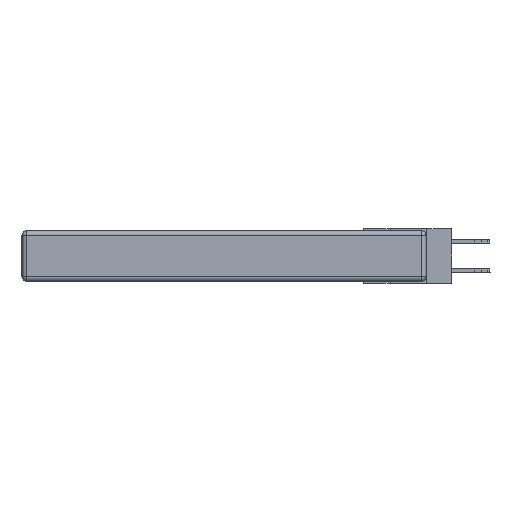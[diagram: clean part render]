
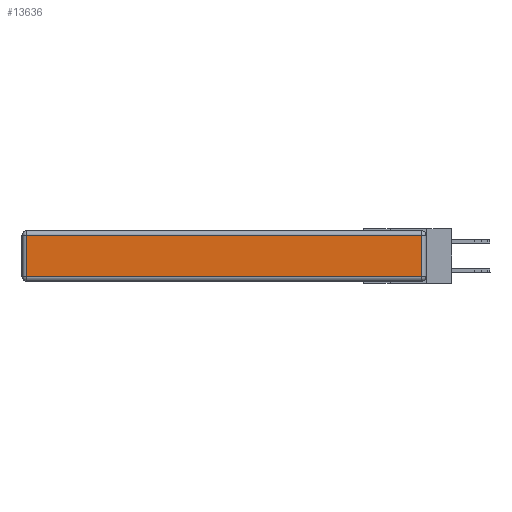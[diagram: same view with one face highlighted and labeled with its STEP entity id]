
A CAD part, left-side view. The second image highlights one B-rep face of the part: STEP entity #13636.
In plain terms, the highlighted planar face has unit normal (-1, 0, 0).
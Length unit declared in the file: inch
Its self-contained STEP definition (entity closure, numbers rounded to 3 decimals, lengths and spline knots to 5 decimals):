
#1110 = CARTESIAN_POINT ( 'NONE',  ( 0., 0.03, -0.313 ) ) ;
#1272 = CARTESIAN_POINT ( 'NONE',  ( 0., 0., -0.343 ) ) ;
#2018 = ORIENTED_EDGE ( 'NONE', *, *, #2638, .T. ) ;
#2610 = VECTOR ( 'NONE', #11376, 39.37008 ) ;
#2638 = EDGE_CURVE ( 'NONE', #4004, #21221, #9904, .T. ) ;
#3493 = VECTOR ( 'NONE', #21026, 39.37008 ) ;
#3643 = CARTESIAN_POINT ( 'NONE',  ( 0., 2.72, -0.313 ) ) ;
#4004 = VERTEX_POINT ( 'NONE', #5706 ) ;
#5398 = AXIS2_PLACEMENT_3D ( 'NONE', #1272, #11630, #13740 ) ;
#5706 = CARTESIAN_POINT ( 'NONE',  ( 0., 0.03, -0.03 ) ) ;
#6139 = DIRECTION ( 'NONE',  ( 0., -1., 0. ) ) ;
#6244 = PLANE ( 'NONE',  #5398 ) ;
#8753 = CARTESIAN_POINT ( 'NONE',  ( 0., 2.72, -0.03 ) ) ;
#9904 = LINE ( 'NONE', #11605, #2610 ) ;
#9993 = LINE ( 'NONE', #13917, #16485 ) ;
#10216 = LINE ( 'NONE', #13760, #3493 ) ;
#10365 = EDGE_LOOP ( 'NONE', ( #19891, #15674, #2018, #19196 ) ) ;
#10647 = FACE_OUTER_BOUND ( 'NONE', #10365, .T. ) ;
#11045 = LINE ( 'NONE', #13548, #17545 ) ;
#11376 = DIRECTION ( 'NONE',  ( 0., 1., 0. ) ) ;
#11605 = CARTESIAN_POINT ( 'NONE',  ( 0., 2.75, -0.03 ) ) ;
#11630 = DIRECTION ( 'NONE',  ( -1., 0., 0. ) ) ;
#11913 = EDGE_CURVE ( 'NONE', #21221, #13949, #10216, .T. ) ;
#12049 = DIRECTION ( 'NONE',  ( 0., 0., 1. ) ) ;
#12522 = EDGE_CURVE ( 'NONE', #13949, #19612, #11045, .T. ) ;
#13548 = CARTESIAN_POINT ( 'NONE',  ( 0., 0., -0.313 ) ) ;
#13636 = ADVANCED_FACE ( 'NONE', ( #10647 ), #6244, .T. ) ;
#13740 = DIRECTION ( 'NONE',  ( 0., 0., 1. ) ) ;
#13760 = CARTESIAN_POINT ( 'NONE',  ( 0., 2.72, -0.343 ) ) ;
#13917 = CARTESIAN_POINT ( 'NONE',  ( 0., 0.03, -0.343 ) ) ;
#13949 = VERTEX_POINT ( 'NONE', #3643 ) ;
#15507 = EDGE_CURVE ( 'NONE', #19612, #4004, #9993, .T. ) ;
#15674 = ORIENTED_EDGE ( 'NONE', *, *, #15507, .T. ) ;
#16485 = VECTOR ( 'NONE', #12049, 39.37008 ) ;
#17545 = VECTOR ( 'NONE', #6139, 39.37008 ) ;
#19196 = ORIENTED_EDGE ( 'NONE', *, *, #11913, .T. ) ;
#19612 = VERTEX_POINT ( 'NONE', #1110 ) ;
#19891 = ORIENTED_EDGE ( 'NONE', *, *, #12522, .T. ) ;
#21026 = DIRECTION ( 'NONE',  ( 0., 0., -1. ) ) ;
#21221 = VERTEX_POINT ( 'NONE', #8753 ) ;
